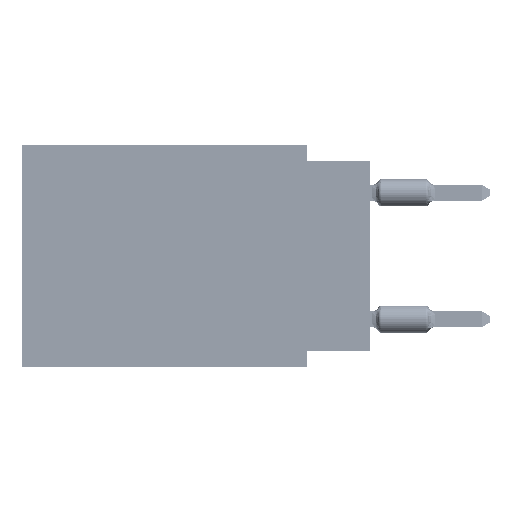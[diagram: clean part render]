
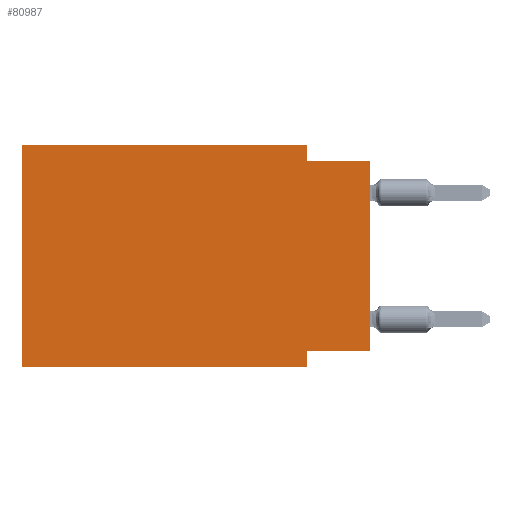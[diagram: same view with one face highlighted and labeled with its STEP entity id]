
A CAD part, left-side view. The second image highlights one B-rep face of the part: STEP entity #80987.
In plain terms, the highlighted planar face has unit normal (-1, 0, 0).
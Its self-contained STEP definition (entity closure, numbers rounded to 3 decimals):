
#1896 = EDGE_CURVE ( 'NONE', #104077, #38837, #104958, .T. ) ;
#5857 = EDGE_CURVE ( 'NONE', #53592, #27207, #24989, .T. ) ;
#8651 = DIRECTION ( 'NONE',  ( 0., -1., 0. ) ) ;
#10165 = ORIENTED_EDGE ( 'NONE', *, *, #1896, .T. ) ;
#10672 = ORIENTED_EDGE ( 'NONE', *, *, #76264, .F. ) ;
#11384 = LINE ( 'NONE', #99037, #52940 ) ;
#12522 = PLANE ( 'NONE',  #89875 ) ;
#13258 = ORIENTED_EDGE ( 'NONE', *, *, #66375, .F. ) ;
#13827 = DIRECTION ( 'NONE',  ( 0., 0., -1. ) ) ;
#17697 = CARTESIAN_POINT ( 'NONE',  ( 0., 0., -0.635 ) ) ;
#17800 = VERTEX_POINT ( 'NONE', #71182 ) ;
#17897 = DIRECTION ( 'NONE',  ( 0., 0., 1. ) ) ;
#18127 = VECTOR ( 'NONE', #8651, 1000. ) ;
#21194 = FACE_OUTER_BOUND ( 'NONE', #59512, .T. ) ;
#21793 = VECTOR ( 'NONE', #113607, 1000. ) ;
#22127 = EDGE_CURVE ( 'NONE', #57944, #27207, #84801, .T. ) ;
#22331 = DIRECTION ( 'NONE',  ( 0., 0., -1. ) ) ;
#24989 = LINE ( 'NONE', #34765, #40190 ) ;
#25295 = EDGE_CURVE ( 'NONE', #48471, #57944, #66872, .T. ) ;
#27207 = VERTEX_POINT ( 'NONE', #17697 ) ;
#28581 = DIRECTION ( 'NONE',  ( 0., -1., 0. ) ) ;
#31830 = CARTESIAN_POINT ( 'NONE',  ( 0., 13.97, -8.89 ) ) ;
#32229 = CARTESIAN_POINT ( 'NONE',  ( 0., 13.97, 0. ) ) ;
#34151 = VECTOR ( 'NONE', #17897, 1000. ) ;
#34765 = CARTESIAN_POINT ( 'NONE',  ( 0., 0., 0. ) ) ;
#38837 = VERTEX_POINT ( 'NONE', #58297 ) ;
#40190 = VECTOR ( 'NONE', #52627, 1000. ) ;
#46569 = DIRECTION ( 'NONE',  ( 0., 0., -1. ) ) ;
#48471 = VERTEX_POINT ( 'NONE', #71839 ) ;
#52627 = DIRECTION ( 'NONE',  ( 0., 0., 1. ) ) ;
#52940 = VECTOR ( 'NONE', #46569, 1000. ) ;
#53592 = VERTEX_POINT ( 'NONE', #60631 ) ;
#54424 = VECTOR ( 'NONE', #101627, 1000. ) ;
#57944 = VERTEX_POINT ( 'NONE', #87061 ) ;
#58297 = CARTESIAN_POINT ( 'NONE',  ( 0., 2.54, -8.89 ) ) ;
#59512 = EDGE_LOOP ( 'NONE', ( #104933, #63887, #76299, #77719, #13258, #10165, #111308, #10672 ) ) ;
#60631 = CARTESIAN_POINT ( 'NONE',  ( 0., 0., -8.255 ) ) ;
#62035 = CARTESIAN_POINT ( 'NONE',  ( 0., 13.97, 0. ) ) ;
#63887 = ORIENTED_EDGE ( 'NONE', *, *, #22127, .F. ) ;
#64445 = CARTESIAN_POINT ( 'NONE',  ( 0., 13.97, 0. ) ) ;
#66144 = DIRECTION ( 'NONE',  ( 1., 0., 0. ) ) ;
#66375 = EDGE_CURVE ( 'NONE', #104077, #66623, #112495, .T. ) ;
#66623 = VERTEX_POINT ( 'NONE', #32229 ) ;
#66872 = LINE ( 'NONE', #84736, #103481 ) ;
#67225 = VECTOR ( 'NONE', #28581, 1000. ) ;
#71182 = CARTESIAN_POINT ( 'NONE',  ( 0., 2.54, -8.255 ) ) ;
#71839 = CARTESIAN_POINT ( 'NONE',  ( 0., 2.54, 0. ) ) ;
#76264 = EDGE_CURVE ( 'NONE', #53592, #17800, #101071, .T. ) ;
#76299 = ORIENTED_EDGE ( 'NONE', *, *, #25295, .F. ) ;
#77719 = ORIENTED_EDGE ( 'NONE', *, *, #108456, .F. ) ;
#78448 = CARTESIAN_POINT ( 'NONE',  ( 0., 0., -0.635 ) ) ;
#80987 = ADVANCED_FACE ( 'NONE', ( #21194 ), #12522, .F. ) ;
#84736 = CARTESIAN_POINT ( 'NONE',  ( 0., 2.54, 0. ) ) ;
#84801 = LINE ( 'NONE', #78448, #21793 ) ;
#87061 = CARTESIAN_POINT ( 'NONE',  ( 0., 2.54, -0.635 ) ) ;
#89522 = EDGE_CURVE ( 'NONE', #17800, #38837, #11384, .T. ) ;
#89875 = AXIS2_PLACEMENT_3D ( 'NONE', #64445, #66144, #22331 ) ;
#96860 = CARTESIAN_POINT ( 'NONE',  ( 0., 13.97, -8.89 ) ) ;
#99037 = CARTESIAN_POINT ( 'NONE',  ( 0., 2.54, -8.89 ) ) ;
#101071 = LINE ( 'NONE', #102200, #54424 ) ;
#101627 = DIRECTION ( 'NONE',  ( 0., 1., 0. ) ) ;
#102200 = CARTESIAN_POINT ( 'NONE',  ( 0., 0., -8.255 ) ) ;
#103481 = VECTOR ( 'NONE', #13827, 1000. ) ;
#104077 = VERTEX_POINT ( 'NONE', #31830 ) ;
#104933 = ORIENTED_EDGE ( 'NONE', *, *, #5857, .T. ) ;
#104958 = LINE ( 'NONE', #96860, #18127 ) ;
#107556 = LINE ( 'NONE', #62035, #67225 ) ;
#108456 = EDGE_CURVE ( 'NONE', #66623, #48471, #107556, .T. ) ;
#111308 = ORIENTED_EDGE ( 'NONE', *, *, #89522, .F. ) ;
#112495 = LINE ( 'NONE', #113632, #34151 ) ;
#113607 = DIRECTION ( 'NONE',  ( 0., -1., 0. ) ) ;
#113632 = CARTESIAN_POINT ( 'NONE',  ( 0., 13.97, 0. ) ) ;
